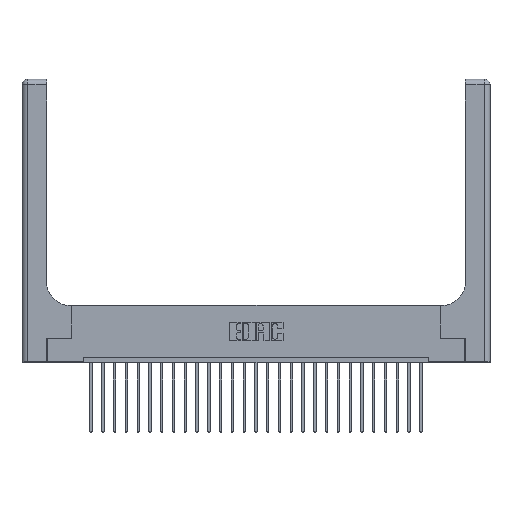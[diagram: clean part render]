
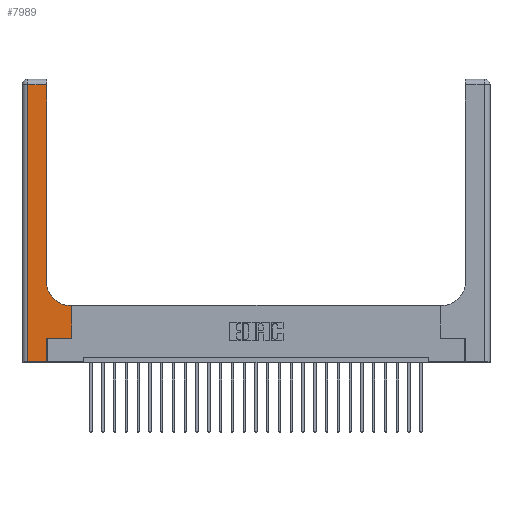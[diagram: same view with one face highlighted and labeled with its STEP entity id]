
A CAD part, top view. The second image highlights one B-rep face of the part: STEP entity #7989.
In plain terms, the highlighted planar face has unit normal (0, 0, 1).
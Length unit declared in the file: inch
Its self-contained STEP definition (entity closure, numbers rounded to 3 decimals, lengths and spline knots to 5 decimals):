
#230 = EDGE_CURVE ( 'NONE', #17480, #19142, #21771, .T. ) ;
#239 = ORIENTED_EDGE ( 'NONE', *, *, #2630, .T. ) ;
#328 = EDGE_CURVE ( 'NONE', #19035, #14060, #12411, .T. ) ;
#347 = VECTOR ( 'NONE', #6311, 39.37008 ) ;
#406 = EDGE_CURVE ( 'NONE', #14060, #8367, #6068, .T. ) ;
#515 = CARTESIAN_POINT ( 'NONE',  ( 0., 2.94, 0.37 ) ) ;
#1007 = CARTESIAN_POINT ( 'NONE',  ( 0.26, 0.6, 0.37 ) ) ;
#1051 = CARTESIAN_POINT ( 'NONE',  ( 0.265, 0., 0.37 ) ) ;
#1161 = LINE ( 'NONE', #1007, #1482 ) ;
#1477 = CARTESIAN_POINT ( 'NONE',  ( 0.06, 0., 0.37 ) ) ;
#1482 = VECTOR ( 'NONE', #22276, 39.37008 ) ;
#2156 = AXIS2_PLACEMENT_3D ( 'NONE', #12136, #21770, #18163 ) ;
#2329 = VECTOR ( 'NONE', #16785, 39.37008 ) ;
#2630 = EDGE_CURVE ( 'NONE', #8367, #22189, #10691, .T. ) ;
#3592 = LINE ( 'NONE', #14082, #17786 ) ;
#4545 = DIRECTION ( 'NONE',  ( 1., 0., 0. ) ) ;
#6017 = ORIENTED_EDGE ( 'NONE', *, *, #24912, .T. ) ;
#6068 = LINE ( 'NONE', #515, #347 ) ;
#6148 = ORIENTED_EDGE ( 'NONE', *, *, #21247, .T. ) ;
#6311 = DIRECTION ( 'NONE',  ( -1., 0., 0. ) ) ;
#6669 = EDGE_CURVE ( 'NONE', #11413, #16371, #3592, .T. ) ;
#6966 = CARTESIAN_POINT ( 'NONE',  ( 0.26, 2.94, 0.37 ) ) ;
#7233 = ORIENTED_EDGE ( 'NONE', *, *, #6669, .T. ) ;
#7351 = CARTESIAN_POINT ( 'NONE',  ( 0.26, 3., 0.37 ) ) ;
#7942 = CARTESIAN_POINT ( 'NONE',  ( 0.06, 3., 0.37 ) ) ;
#7989 = ADVANCED_FACE ( 'NONE', ( #8054 ), #17109, .F. ) ;
#7997 = LINE ( 'NONE', #19834, #20075 ) ;
#8054 = FACE_OUTER_BOUND ( 'NONE', #8561, .T. ) ;
#8367 = VERTEX_POINT ( 'NONE', #17107 ) ;
#8561 = EDGE_LOOP ( 'NONE', ( #20038, #11193, #239, #23133, #9703, #18243, #7233, #6148, #6017 ) ) ;
#9703 = ORIENTED_EDGE ( 'NONE', *, *, #230, .T. ) ;
#10533 = AXIS2_PLACEMENT_3D ( 'NONE', #13355, #17275, #19282 ) ;
#10691 = LINE ( 'NONE', #7942, #12203 ) ;
#10848 = CARTESIAN_POINT ( 'NONE',  ( 0., 0., 0.37 ) ) ;
#11193 = ORIENTED_EDGE ( 'NONE', *, *, #406, .T. ) ;
#11413 = VERTEX_POINT ( 'NONE', #17269 ) ;
#12090 = VECTOR ( 'NONE', #20319, 39.37008 ) ;
#12136 = CARTESIAN_POINT ( 'NONE',  ( 0.51, 0.85, 0.37 ) ) ;
#12155 = CARTESIAN_POINT ( 'NONE',  ( 0.26, 0.85, 0.37 ) ) ;
#12203 = VECTOR ( 'NONE', #13919, 39.37008 ) ;
#12411 = LINE ( 'NONE', #7351, #16046 ) ;
#12453 = CARTESIAN_POINT ( 'NONE',  ( 0.265, 0., 0.37 ) ) ;
#13355 = CARTESIAN_POINT ( 'NONE',  ( 0., 3., 0.37 ) ) ;
#13919 = DIRECTION ( 'NONE',  ( 0., -1., 0. ) ) ;
#14060 = VERTEX_POINT ( 'NONE', #6966 ) ;
#14082 = CARTESIAN_POINT ( 'NONE',  ( 0.528, 0.25, 0.37 ) ) ;
#14772 = CARTESIAN_POINT ( 'NONE',  ( 0.265, 0.25, 0.37 ) ) ;
#15317 = CARTESIAN_POINT ( 'NONE',  ( 0.51, 0.6, 0.37 ) ) ;
#15720 = DIRECTION ( 'NONE',  ( 0., 1., 0. ) ) ;
#16046 = VECTOR ( 'NONE', #15720, 39.37008 ) ;
#16371 = VERTEX_POINT ( 'NONE', #23308 ) ;
#16785 = DIRECTION ( 'NONE',  ( 1., 0., 0. ) ) ;
#17015 = EDGE_CURVE ( 'NONE', #19142, #11413, #7997, .T. ) ;
#17107 = CARTESIAN_POINT ( 'NONE',  ( 0.06, 2.94, 0.37 ) ) ;
#17109 = PLANE ( 'NONE',  #10533 ) ;
#17269 = CARTESIAN_POINT ( 'NONE',  ( 0.528, 0.25, 0.37 ) ) ;
#17275 = DIRECTION ( 'NONE',  ( 0., 0., -1. ) ) ;
#17480 = VERTEX_POINT ( 'NONE', #1051 ) ;
#17786 = VECTOR ( 'NONE', #18011, 39.37008 ) ;
#18011 = DIRECTION ( 'NONE',  ( 0., 1., 0. ) ) ;
#18061 = LINE ( 'NONE', #10848, #2329 ) ;
#18163 = DIRECTION ( 'NONE',  ( 1., 0., 0. ) ) ;
#18243 = ORIENTED_EDGE ( 'NONE', *, *, #17015, .T. ) ;
#19035 = VERTEX_POINT ( 'NONE', #12155 ) ;
#19142 = VERTEX_POINT ( 'NONE', #14772 ) ;
#19203 = CIRCLE ( 'NONE', #2156, 0.25 ) ;
#19282 = DIRECTION ( 'NONE',  ( -1., 0., 0. ) ) ;
#19834 = CARTESIAN_POINT ( 'NONE',  ( 0.265, 0.25, 0.37 ) ) ;
#20038 = ORIENTED_EDGE ( 'NONE', *, *, #328, .T. ) ;
#20075 = VECTOR ( 'NONE', #4545, 39.37008 ) ;
#20319 = DIRECTION ( 'NONE',  ( 0., 1., 0. ) ) ;
#21247 = EDGE_CURVE ( 'NONE', #16371, #21965, #1161, .T. ) ;
#21770 = DIRECTION ( 'NONE',  ( 0., 0., -1. ) ) ;
#21771 = LINE ( 'NONE', #12453, #12090 ) ;
#21965 = VERTEX_POINT ( 'NONE', #15317 ) ;
#22189 = VERTEX_POINT ( 'NONE', #1477 ) ;
#22276 = DIRECTION ( 'NONE',  ( -1., 0., 0. ) ) ;
#23133 = ORIENTED_EDGE ( 'NONE', *, *, #23524, .T. ) ;
#23308 = CARTESIAN_POINT ( 'NONE',  ( 0.528, 0.6, 0.37 ) ) ;
#23524 = EDGE_CURVE ( 'NONE', #22189, #17480, #18061, .T. ) ;
#24912 = EDGE_CURVE ( 'NONE', #21965, #19035, #19203, .T. ) ;
